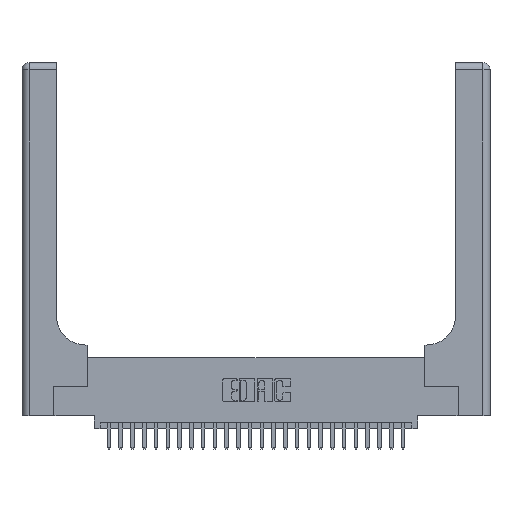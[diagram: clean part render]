
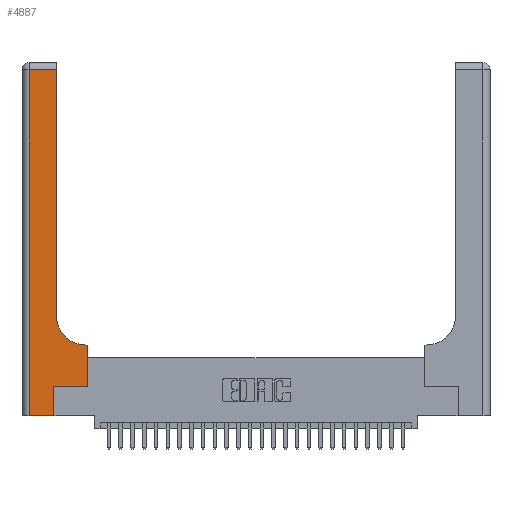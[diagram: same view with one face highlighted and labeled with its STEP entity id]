
A CAD part, top view. The second image highlights one B-rep face of the part: STEP entity #4887.
In plain terms, the highlighted planar face has unit normal (0, 0, 1).
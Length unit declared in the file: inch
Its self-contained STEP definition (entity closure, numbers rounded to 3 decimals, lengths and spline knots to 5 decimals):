
#85 = DIRECTION ( 'NONE',  ( 0., 1., 0. ) ) ;
#645 = DIRECTION ( 'NONE',  ( -1., 0., 0. ) ) ;
#1421 = VERTEX_POINT ( 'NONE', #10027 ) ;
#1666 = ORIENTED_EDGE ( 'NONE', *, *, #9622, .T. ) ;
#2650 = VERTEX_POINT ( 'NONE', #20239 ) ;
#2692 = CARTESIAN_POINT ( 'NONE',  ( 0.269, 0., 0.37 ) ) ;
#3354 = LINE ( 'NONE', #12199, #20534 ) ;
#3446 = ORIENTED_EDGE ( 'NONE', *, *, #11281, .T. ) ;
#3641 = DIRECTION ( 'NONE',  ( -1., 0., 0. ) ) ;
#3743 = CARTESIAN_POINT ( 'NONE',  ( 0.2915, 2.94, 0.37 ) ) ;
#3809 = CARTESIAN_POINT ( 'NONE',  ( 0., 2.94, 0.37 ) ) ;
#4104 = VERTEX_POINT ( 'NONE', #6962 ) ;
#4887 = ADVANCED_FACE ( 'NONE', ( #16654 ), #18521, .F. ) ;
#5070 = LINE ( 'NONE', #2692, #10769 ) ;
#5350 = CARTESIAN_POINT ( 'NONE',  ( 0., 0., 0.37 ) ) ;
#6034 = EDGE_LOOP ( 'NONE', ( #25663, #24481, #16019, #15407, #18673, #25231, #13146, #3446, #1666 ) ) ;
#6072 = AXIS2_PLACEMENT_3D ( 'NONE', #13879, #26939, #18212 ) ;
#6962 = CARTESIAN_POINT ( 'NONE',  ( 0.2915, 0.85, 0.37 ) ) ;
#9622 = EDGE_CURVE ( 'NONE', #17566, #4104, #16680, .T. ) ;
#9952 = DIRECTION ( 'NONE',  ( 0., -1., 0. ) ) ;
#10027 = CARTESIAN_POINT ( 'NONE',  ( 0.06, 2.94, 0.37 ) ) ;
#10769 = VECTOR ( 'NONE', #22238, 39.37008 ) ;
#10915 = LINE ( 'NONE', #17507, #19410 ) ;
#11281 = EDGE_CURVE ( 'NONE', #20990, #17566, #17237, .T. ) ;
#11994 = EDGE_CURVE ( 'NONE', #2650, #19149, #5070, .T. ) ;
#12091 = CARTESIAN_POINT ( 'NONE',  ( 0., 3., 0.37 ) ) ;
#12199 = CARTESIAN_POINT ( 'NONE',  ( 0.2915, 3., 0.37 ) ) ;
#12212 = CARTESIAN_POINT ( 'NONE',  ( 0.06, 0., 0.37 ) ) ;
#13099 = VECTOR ( 'NONE', #20517, 39.37008 ) ;
#13146 = ORIENTED_EDGE ( 'NONE', *, *, #21559, .T. ) ;
#13175 = EDGE_CURVE ( 'NONE', #4104, #18241, #3354, .T. ) ;
#13879 = CARTESIAN_POINT ( 'NONE',  ( 0.5415, 0.85, 0.37 ) ) ;
#14174 = VECTOR ( 'NONE', #23612, 39.37008 ) ;
#15407 = ORIENTED_EDGE ( 'NONE', *, *, #17970, .T. ) ;
#16019 = ORIENTED_EDGE ( 'NONE', *, *, #23006, .T. ) ;
#16299 = CARTESIAN_POINT ( 'NONE',  ( 0.06, 3., 0.37 ) ) ;
#16654 = FACE_OUTER_BOUND ( 'NONE', #6034, .T. ) ;
#16680 = CIRCLE ( 'NONE', #6072, 0.25 ) ;
#17237 = LINE ( 'NONE', #26334, #22348 ) ;
#17247 = CARTESIAN_POINT ( 'NONE',  ( 0.269, 0.25, 0.37 ) ) ;
#17347 = CARTESIAN_POINT ( 'NONE',  ( 0.5585, 0.25, 0.37 ) ) ;
#17507 = CARTESIAN_POINT ( 'NONE',  ( 0.5585, 0.25, 0.37 ) ) ;
#17537 = CARTESIAN_POINT ( 'NONE',  ( 0.269, 0.25, 0.37 ) ) ;
#17566 = VERTEX_POINT ( 'NONE', #23003 ) ;
#17970 = EDGE_CURVE ( 'NONE', #18201, #2650, #25301, .T. ) ;
#18201 = VERTEX_POINT ( 'NONE', #12212 ) ;
#18212 = DIRECTION ( 'NONE',  ( 1., 0., 0. ) ) ;
#18241 = VERTEX_POINT ( 'NONE', #3743 ) ;
#18521 = PLANE ( 'NONE',  #25706 ) ;
#18673 = ORIENTED_EDGE ( 'NONE', *, *, #11994, .T. ) ;
#18734 = DIRECTION ( 'NONE',  ( -1., 0., 0. ) ) ;
#19149 = VERTEX_POINT ( 'NONE', #17537 ) ;
#19259 = VECTOR ( 'NONE', #3641, 39.37008 ) ;
#19410 = VECTOR ( 'NONE', #85, 39.37008 ) ;
#19559 = CARTESIAN_POINT ( 'NONE',  ( 0.5585, 0.6, 0.37 ) ) ;
#19694 = DIRECTION ( 'NONE',  ( 0., 0., -1. ) ) ;
#20239 = CARTESIAN_POINT ( 'NONE',  ( 0.269, 0., 0.37 ) ) ;
#20517 = DIRECTION ( 'NONE',  ( 1., 0., 0. ) ) ;
#20534 = VECTOR ( 'NONE', #24961, 39.37008 ) ;
#20990 = VERTEX_POINT ( 'NONE', #19559 ) ;
#21559 = EDGE_CURVE ( 'NONE', #26883, #20990, #10915, .T. ) ;
#22238 = DIRECTION ( 'NONE',  ( 0., 1., 0. ) ) ;
#22348 = VECTOR ( 'NONE', #645, 39.37008 ) ;
#23003 = CARTESIAN_POINT ( 'NONE',  ( 0.5415, 0.6, 0.37 ) ) ;
#23006 = EDGE_CURVE ( 'NONE', #1421, #18201, #23770, .T. ) ;
#23612 = DIRECTION ( 'NONE',  ( 1., 0., 0. ) ) ;
#23770 = LINE ( 'NONE', #16299, #26125 ) ;
#24481 = ORIENTED_EDGE ( 'NONE', *, *, #25076, .T. ) ;
#24961 = DIRECTION ( 'NONE',  ( 0., 1., 0. ) ) ;
#25076 = EDGE_CURVE ( 'NONE', #18241, #1421, #27740, .T. ) ;
#25231 = ORIENTED_EDGE ( 'NONE', *, *, #25258, .T. ) ;
#25258 = EDGE_CURVE ( 'NONE', #19149, #26883, #25690, .T. ) ;
#25301 = LINE ( 'NONE', #5350, #13099 ) ;
#25663 = ORIENTED_EDGE ( 'NONE', *, *, #13175, .T. ) ;
#25690 = LINE ( 'NONE', #17247, #14174 ) ;
#25706 = AXIS2_PLACEMENT_3D ( 'NONE', #12091, #19694, #18734 ) ;
#26125 = VECTOR ( 'NONE', #9952, 39.37008 ) ;
#26334 = CARTESIAN_POINT ( 'NONE',  ( 0.2915, 0.6, 0.37 ) ) ;
#26883 = VERTEX_POINT ( 'NONE', #17347 ) ;
#26939 = DIRECTION ( 'NONE',  ( 0., 0., -1. ) ) ;
#27740 = LINE ( 'NONE', #3809, #19259 ) ;
